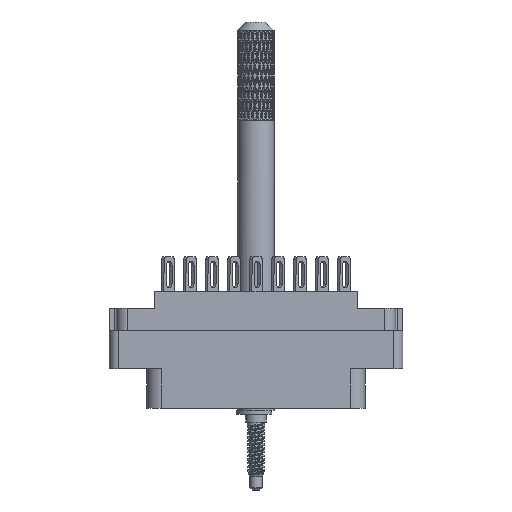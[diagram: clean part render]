
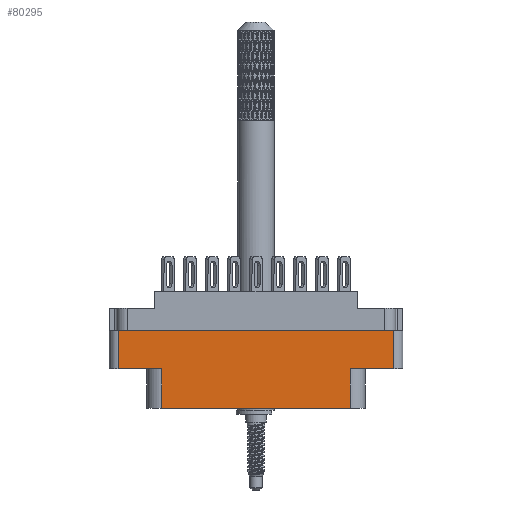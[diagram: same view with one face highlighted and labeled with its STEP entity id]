
A CAD part, front view. The second image highlights one B-rep face of the part: STEP entity #80295.
In plain terms, the highlighted planar face has unit normal (0, -1, 0).
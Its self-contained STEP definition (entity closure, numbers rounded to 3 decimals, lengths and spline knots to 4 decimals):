
#3582 = VECTOR ( 'NONE', #75719, 39.3701 ) ;
#3865 = VECTOR ( 'NONE', #14601, 39.3701 ) ;
#3907 = ORIENTED_EDGE ( 'NONE', *, *, #37667, .T. ) ;
#4277 = EDGE_CURVE ( 'NONE', #15415, #8316, #29705, .T. ) ;
#4585 = EDGE_CURVE ( 'NONE', #26029, #52802, #40787, .T. ) ;
#7410 = CARTESIAN_POINT ( 'NONE',  ( -0.938, -0.438, -0.798 ) ) ;
#8316 = VERTEX_POINT ( 'NONE', #29465 ) ;
#9216 = LINE ( 'NONE', #94331, #41153 ) ;
#12783 = EDGE_CURVE ( 'NONE', #16553, #52802, #87581, .T. ) ;
#14358 = DIRECTION ( 'NONE',  ( 0., 0., -1. ) ) ;
#14601 = DIRECTION ( 'NONE',  ( 0., 0., -1. ) ) ;
#15415 = VERTEX_POINT ( 'NONE', #96788 ) ;
#16553 = VERTEX_POINT ( 'NONE', #62784 ) ;
#19847 = EDGE_CURVE ( 'NONE', #16553, #59360, #82425, .T. ) ;
#22623 = DIRECTION ( 'NONE',  ( 0., -1., 0. ) ) ;
#26029 = VERTEX_POINT ( 'NONE', #95583 ) ;
#29252 = VECTOR ( 'NONE', #90061, 39.3701 ) ;
#29465 = CARTESIAN_POINT ( 'NONE',  ( -0.644, -0.438, -0.798 ) ) ;
#29705 = LINE ( 'NONE', #35535, #87887 ) ;
#34509 = EDGE_CURVE ( 'NONE', #73358, #26029, #68827, .T. ) ;
#34748 = CARTESIAN_POINT ( 'NONE',  ( -0.938, -0.438, -0.798 ) ) ;
#34880 = DIRECTION ( 'NONE',  ( 0., 0., -1. ) ) ;
#35535 = CARTESIAN_POINT ( 'NONE',  ( -0.644, -0.438, -0.529 ) ) ;
#36391 = ORIENTED_EDGE ( 'NONE', *, *, #4585, .F. ) ;
#36417 = CARTESIAN_POINT ( 'NONE',  ( 0., -0.438, -0.529 ) ) ;
#36536 = CARTESIAN_POINT ( 'NONE',  ( -0.938, -0.438, -0.529 ) ) ;
#37667 = EDGE_CURVE ( 'NONE', #73358, #15415, #9216, .T. ) ;
#38437 = CARTESIAN_POINT ( 'NONE',  ( 0.938, -0.438, -0.798 ) ) ;
#38477 = PLANE ( 'NONE',  #76953 ) ;
#38488 = CARTESIAN_POINT ( 'NONE',  ( 0.644, -0.438, -0.529 ) ) ;
#40430 = CARTESIAN_POINT ( 'NONE',  ( 0.938, -0.438, -0.268 ) ) ;
#40787 = LINE ( 'NONE', #73708, #79133 ) ;
#41153 = VECTOR ( 'NONE', #63176, 39.3701 ) ;
#42484 = ORIENTED_EDGE ( 'NONE', *, *, #4277, .T. ) ;
#42785 = VECTOR ( 'NONE', #68236, 39.3701 ) ;
#45616 = ORIENTED_EDGE ( 'NONE', *, *, #19847, .F. ) ;
#48823 = ORIENTED_EDGE ( 'NONE', *, *, #79258, .F. ) ;
#50741 = FACE_OUTER_BOUND ( 'NONE', #71051, .T. ) ;
#52802 = VERTEX_POINT ( 'NONE', #40430 ) ;
#59221 = LINE ( 'NONE', #90938, #3582 ) ;
#59360 = VERTEX_POINT ( 'NONE', #38488 ) ;
#62784 = CARTESIAN_POINT ( 'NONE',  ( 0.938, -0.438, -0.529 ) ) ;
#63176 = DIRECTION ( 'NONE',  ( 1., 0., 0. ) ) ;
#66489 = VECTOR ( 'NONE', #94138, 39.3701 ) ;
#68236 = DIRECTION ( 'NONE',  ( -1., 0., 0. ) ) ;
#68827 = LINE ( 'NONE', #34748, #29252 ) ;
#70181 = CARTESIAN_POINT ( 'NONE',  ( 0.644, -0.438, -0.529 ) ) ;
#71051 = EDGE_LOOP ( 'NONE', ( #42484, #100540, #48823, #45616, #85436, #36391, #92894, #3907 ) ) ;
#71914 = LINE ( 'NONE', #70181, #3865 ) ;
#73358 = VERTEX_POINT ( 'NONE', #36536 ) ;
#73708 = CARTESIAN_POINT ( 'NONE',  ( -1., -0.438, -0.268 ) ) ;
#74682 = CARTESIAN_POINT ( 'NONE',  ( 0.644, -0.438, -0.798 ) ) ;
#75719 = DIRECTION ( 'NONE',  ( 1., 0., 0. ) ) ;
#76953 = AXIS2_PLACEMENT_3D ( 'NONE', #7410, #22623, #14358 ) ;
#79133 = VECTOR ( 'NONE', #85021, 39.3701 ) ;
#79258 = EDGE_CURVE ( 'NONE', #59360, #88696, #71914, .T. ) ;
#80295 = ADVANCED_FACE ( 'NONE', ( #50741 ), #38477, .T. ) ;
#81970 = EDGE_CURVE ( 'NONE', #8316, #88696, #59221, .T. ) ;
#82425 = LINE ( 'NONE', #36417, #42785 ) ;
#85021 = DIRECTION ( 'NONE',  ( 1., 0., 0. ) ) ;
#85436 = ORIENTED_EDGE ( 'NONE', *, *, #12783, .T. ) ;
#87581 = LINE ( 'NONE', #38437, #66489 ) ;
#87887 = VECTOR ( 'NONE', #34880, 39.3701 ) ;
#88696 = VERTEX_POINT ( 'NONE', #74682 ) ;
#90061 = DIRECTION ( 'NONE',  ( 0., 0., 1. ) ) ;
#90938 = CARTESIAN_POINT ( 'NONE',  ( -0.938, -0.438, -0.798 ) ) ;
#92894 = ORIENTED_EDGE ( 'NONE', *, *, #34509, .F. ) ;
#94138 = DIRECTION ( 'NONE',  ( 0., 0., 1. ) ) ;
#94331 = CARTESIAN_POINT ( 'NONE',  ( 0., -0.438, -0.529 ) ) ;
#95583 = CARTESIAN_POINT ( 'NONE',  ( -0.938, -0.438, -0.268 ) ) ;
#96788 = CARTESIAN_POINT ( 'NONE',  ( -0.644, -0.438, -0.529 ) ) ;
#100540 = ORIENTED_EDGE ( 'NONE', *, *, #81970, .T. ) ;
